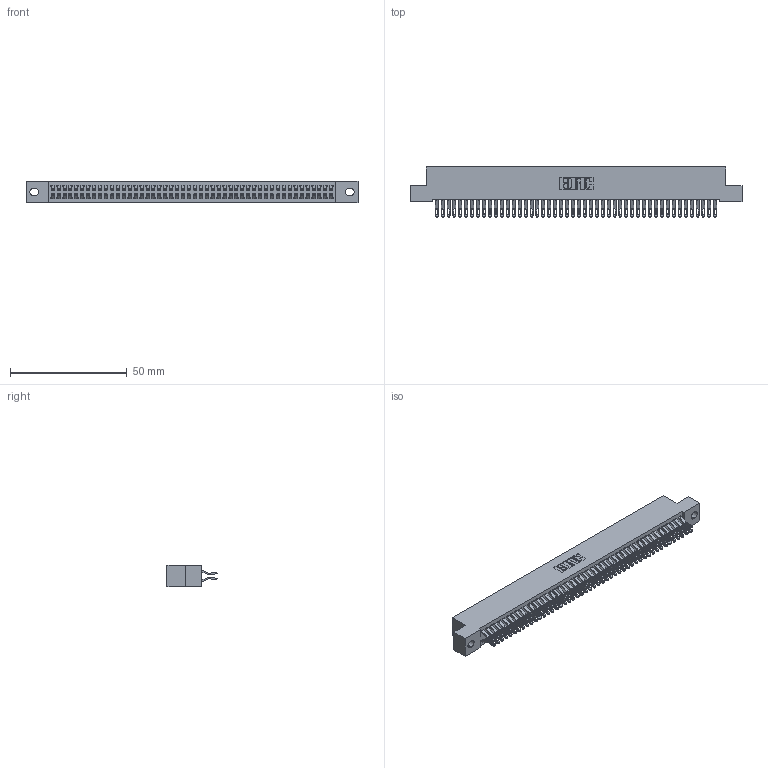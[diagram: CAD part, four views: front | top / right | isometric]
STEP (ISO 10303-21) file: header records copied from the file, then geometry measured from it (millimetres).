
FILE_DESCRIPTION (( 'STEP AP203' ), '1' );
FILE_NAME ('342-096-555-202.STEP', '2018-08-14T03:19:34', ( '' ), ( '' ), 'SwSTEP 2.0', 'SolidWorks 2016', '' );
FILE_SCHEMA (( 'CONFIG_CONTROL_DESIGN' ));
Length unit declared in the file: inch
Products named in the file (3): 342 Part_.128 Slot; 345-292-001_555 Tail; 342-096-555-202
Assembly tree (97 placements, depth 2):
  342-096-555-202
    342 Part_.128 Slot
    345-292-001_555 Tail  x96
Bounding box: 142.24 x 21.47 x 9.4 mm (x, y, z)
Volume: 13023.3 mm3; surface area: 22034.8 mm2
Topology: 97 solids, 97 shells, 5682 faces, 17879 edges, 11918 vertices
Faces by surface type: plane 3334, cylinder 2348
Entity records: 30433 total; most frequent: CARTESIAN_POINT 5072, ORIENTED_EDGE 4978, DIRECTION 4293, EDGE_CURVE 2489, VECTOR 2341, LINE 2341, VERTEX_POINT 1658, AXIS2_PLACEMENT_3D 976
